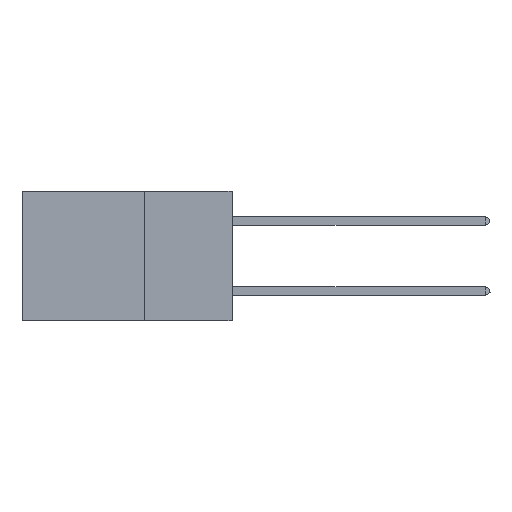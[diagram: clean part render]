
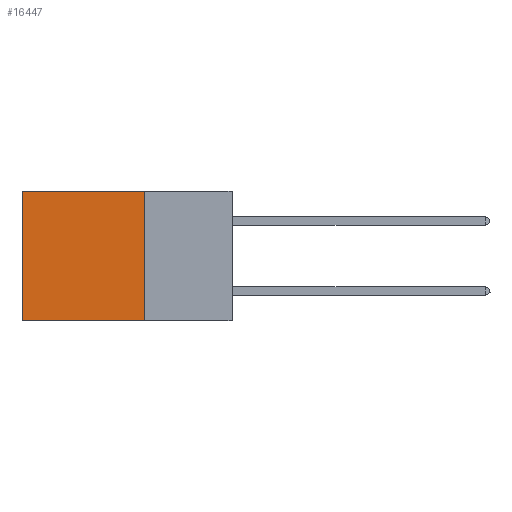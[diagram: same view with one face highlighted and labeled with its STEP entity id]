
A CAD part, left-side view. The second image highlights one B-rep face of the part: STEP entity #16447.
In plain terms, the highlighted planar face has unit normal (-1, 0, 0).
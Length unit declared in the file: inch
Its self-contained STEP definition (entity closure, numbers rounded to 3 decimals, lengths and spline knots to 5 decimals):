
#1151 = EDGE_CURVE ( 'NONE', #1740, #1651, #25192, .T. ) ;
#1414 = LINE ( 'NONE', #6539, #28254 ) ;
#1651 = VERTEX_POINT ( 'NONE', #14427 ) ;
#1740 = VERTEX_POINT ( 'NONE', #10892 ) ;
#3032 = VERTEX_POINT ( 'NONE', #14200 ) ;
#4067 = ORIENTED_EDGE ( 'NONE', *, *, #19447, .F. ) ;
#6099 = CARTESIAN_POINT ( 'NONE',  ( 0.2875, 0.6, -0.37 ) ) ;
#6539 = CARTESIAN_POINT ( 'NONE',  ( 0.2875, 0.6, 0. ) ) ;
#8689 = ORIENTED_EDGE ( 'NONE', *, *, #25893, .T. ) ;
#8905 = VERTEX_POINT ( 'NONE', #6099 ) ;
#9023 = DIRECTION ( 'NONE',  ( 0., 0., -1. ) ) ;
#9297 = VECTOR ( 'NONE', #16282, 39.37008 ) ;
#10573 = LINE ( 'NONE', #22528, #26531 ) ;
#10892 = CARTESIAN_POINT ( 'NONE',  ( 0.2875, 0.25, 0. ) ) ;
#12154 = DIRECTION ( 'NONE',  ( 0., 1., 0. ) ) ;
#12509 = DIRECTION ( 'NONE',  ( 0., 0., -1. ) ) ;
#12830 = CARTESIAN_POINT ( 'NONE',  ( 0.2875, 0.25, 0. ) ) ;
#14200 = CARTESIAN_POINT ( 'NONE',  ( 0.2875, 0.25, -0.37 ) ) ;
#14427 = CARTESIAN_POINT ( 'NONE',  ( 0.2875, 0.6, 0. ) ) ;
#16282 = DIRECTION ( 'NONE',  ( 0., 1., 0. ) ) ;
#16447 = ADVANCED_FACE ( 'NONE', ( #30120 ), #27820, .F. ) ;
#19392 = ORIENTED_EDGE ( 'NONE', *, *, #1151, .T. ) ;
#19447 = EDGE_CURVE ( 'NONE', #1740, #3032, #10573, .T. ) ;
#21191 = CARTESIAN_POINT ( 'NONE',  ( 0.2875, 0.25, 0. ) ) ;
#22528 = CARTESIAN_POINT ( 'NONE',  ( 0.2875, 0.25, 0. ) ) ;
#22732 = DIRECTION ( 'NONE',  ( 1., 0., 0. ) ) ;
#23262 = VECTOR ( 'NONE', #12154, 39.37008 ) ;
#24390 = ORIENTED_EDGE ( 'NONE', *, *, #27371, .F. ) ;
#24544 = CARTESIAN_POINT ( 'NONE',  ( 0.2875, 0.25, -0.37 ) ) ;
#24949 = EDGE_LOOP ( 'NONE', ( #8689, #24390, #4067, #19392 ) ) ;
#25192 = LINE ( 'NONE', #21191, #9297 ) ;
#25578 = LINE ( 'NONE', #24544, #23262 ) ;
#25660 = DIRECTION ( 'NONE',  ( 0., 0., -1. ) ) ;
#25839 = AXIS2_PLACEMENT_3D ( 'NONE', #12830, #22732, #12509 ) ;
#25893 = EDGE_CURVE ( 'NONE', #1651, #8905, #1414, .T. ) ;
#26531 = VECTOR ( 'NONE', #25660, 39.37008 ) ;
#27371 = EDGE_CURVE ( 'NONE', #3032, #8905, #25578, .T. ) ;
#27820 = PLANE ( 'NONE',  #25839 ) ;
#28254 = VECTOR ( 'NONE', #9023, 39.37008 ) ;
#30120 = FACE_OUTER_BOUND ( 'NONE', #24949, .T. ) ;
